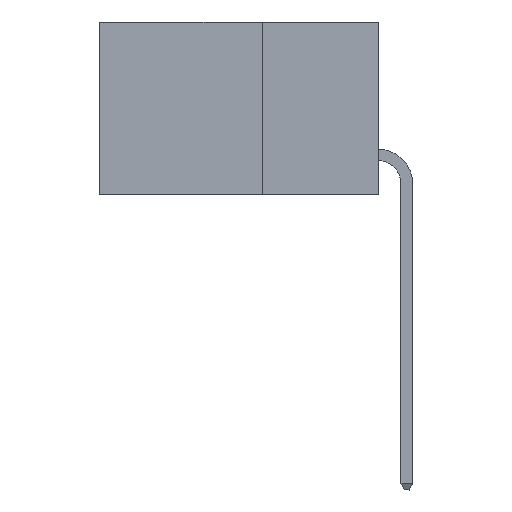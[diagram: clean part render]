
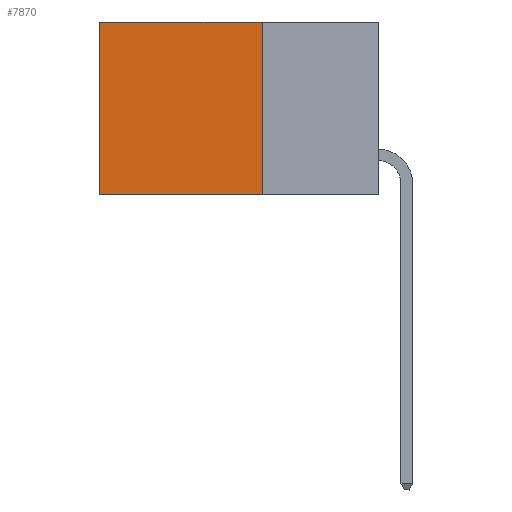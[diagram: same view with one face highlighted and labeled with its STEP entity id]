
A CAD part, left-side view. The second image highlights one B-rep face of the part: STEP entity #7870.
In plain terms, the highlighted planar face has unit normal (-1, 0, 0).
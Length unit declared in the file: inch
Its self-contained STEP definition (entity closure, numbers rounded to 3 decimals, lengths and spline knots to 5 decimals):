
#101 = EDGE_LOOP ( 'NONE', ( #993, #4823, #8538, #4117 ) ) ;
#211 = LINE ( 'NONE', #1417, #5679 ) ;
#993 = ORIENTED_EDGE ( 'NONE', *, *, #3013, .T. ) ;
#1389 = VERTEX_POINT ( 'NONE', #3643 ) ;
#1417 = CARTESIAN_POINT ( 'NONE',  ( 0.298, 0.25, 0. ) ) ;
#1556 = DIRECTION ( 'NONE',  ( 1., 0., 0. ) ) ;
#1854 = VERTEX_POINT ( 'NONE', #6657 ) ;
#1885 = VERTEX_POINT ( 'NONE', #5394 ) ;
#1887 = LINE ( 'NONE', #3586, #5129 ) ;
#2109 = DIRECTION ( 'NONE',  ( 0., 0., -1. ) ) ;
#2617 = EDGE_CURVE ( 'NONE', #1389, #1885, #211, .T. ) ;
#3013 = EDGE_CURVE ( 'NONE', #6921, #1854, #1887, .T. ) ;
#3207 = DIRECTION ( 'NONE',  ( 0., 1., 0. ) ) ;
#3586 = CARTESIAN_POINT ( 'NONE',  ( 0.298, 0.6, 0. ) ) ;
#3643 = CARTESIAN_POINT ( 'NONE',  ( 0.298, 0.25, 0. ) ) ;
#4088 = CARTESIAN_POINT ( 'NONE',  ( 0.298, 0.25, -0.37 ) ) ;
#4117 = ORIENTED_EDGE ( 'NONE', *, *, #8391, .T. ) ;
#4331 = CARTESIAN_POINT ( 'NONE',  ( 0.298, 0.25, 0. ) ) ;
#4377 = EDGE_CURVE ( 'NONE', #1885, #1854, #5295, .T. ) ;
#4823 = ORIENTED_EDGE ( 'NONE', *, *, #4377, .F. ) ;
#5129 = VECTOR ( 'NONE', #2109, 39.37008 ) ;
#5249 = FACE_OUTER_BOUND ( 'NONE', #101, .T. ) ;
#5295 = LINE ( 'NONE', #4088, #5967 ) ;
#5394 = CARTESIAN_POINT ( 'NONE',  ( 0.298, 0.25, -0.37 ) ) ;
#5629 = DIRECTION ( 'NONE',  ( 0., 1., 0. ) ) ;
#5679 = VECTOR ( 'NONE', #7807, 39.37008 ) ;
#5967 = VECTOR ( 'NONE', #5629, 39.37008 ) ;
#5988 = VECTOR ( 'NONE', #3207, 39.37008 ) ;
#5995 = AXIS2_PLACEMENT_3D ( 'NONE', #4331, #1556, #8543 ) ;
#6347 = CARTESIAN_POINT ( 'NONE',  ( 0.298, 0.6, 0. ) ) ;
#6657 = CARTESIAN_POINT ( 'NONE',  ( 0.298, 0.6, -0.37 ) ) ;
#6921 = VERTEX_POINT ( 'NONE', #6347 ) ;
#7134 = PLANE ( 'NONE',  #5995 ) ;
#7244 = CARTESIAN_POINT ( 'NONE',  ( 0.298, 0.25, 0. ) ) ;
#7807 = DIRECTION ( 'NONE',  ( 0., 0., -1. ) ) ;
#7870 = ADVANCED_FACE ( 'NONE', ( #5249 ), #7134, .F. ) ;
#7898 = LINE ( 'NONE', #7244, #5988 ) ;
#8391 = EDGE_CURVE ( 'NONE', #1389, #6921, #7898, .T. ) ;
#8538 = ORIENTED_EDGE ( 'NONE', *, *, #2617, .F. ) ;
#8543 = DIRECTION ( 'NONE',  ( 0., 0., -1. ) ) ;
